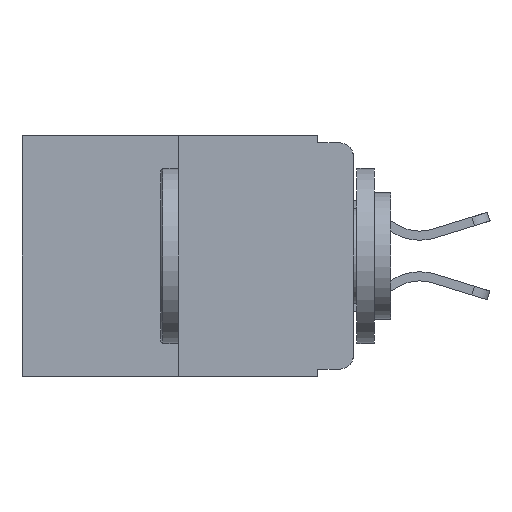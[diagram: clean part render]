
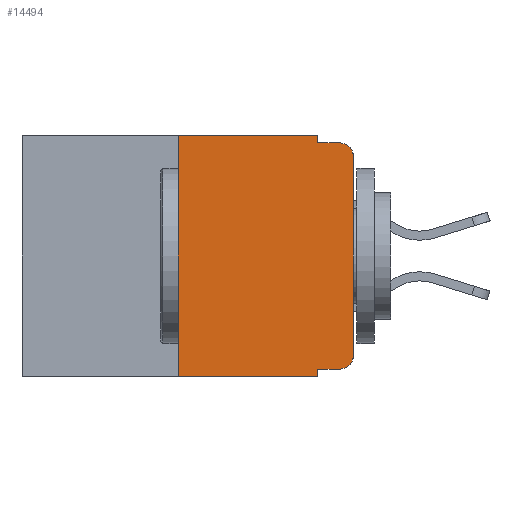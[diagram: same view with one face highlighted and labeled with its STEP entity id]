
A CAD part, left-side view. The second image highlights one B-rep face of the part: STEP entity #14494.
In plain terms, the highlighted planar face has unit normal (-1, 0, 0).
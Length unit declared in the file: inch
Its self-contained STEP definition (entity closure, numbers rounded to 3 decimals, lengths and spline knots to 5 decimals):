
#337 = CARTESIAN_POINT ( 'NONE',  ( 0., 0.473, 0. ) ) ;
#623 = DIRECTION ( 'NONE',  ( 0., -1., 0. ) ) ;
#686 = LINE ( 'NONE', #337, #7362 ) ;
#712 = EDGE_CURVE ( 'NONE', #9476, #1143, #9028, .T. ) ;
#891 = CARTESIAN_POINT ( 'NONE',  ( 0., 0.02, -0.03 ) ) ;
#1072 = VECTOR ( 'NONE', #5682, 39.37008 ) ;
#1143 = VERTEX_POINT ( 'NONE', #4148 ) ;
#1169 = CARTESIAN_POINT ( 'NONE',  ( 0., 0.051, 0. ) ) ;
#1214 = CARTESIAN_POINT ( 'NONE',  ( 0., 0.051, -0.333 ) ) ;
#1677 = CARTESIAN_POINT ( 'NONE',  ( 0., 0.473, 0. ) ) ;
#1696 = CIRCLE ( 'NONE', #11862, 0.02 ) ;
#1710 = DIRECTION ( 'NONE',  ( 0., 0., -1. ) ) ;
#2031 = LINE ( 'NONE', #1214, #5386 ) ;
#2071 = FACE_OUTER_BOUND ( 'NONE', #13560, .T. ) ;
#2201 = DIRECTION ( 'NONE',  ( 0., 0., -1. ) ) ;
#2268 = LINE ( 'NONE', #1169, #14534 ) ;
#2578 = ORIENTED_EDGE ( 'NONE', *, *, #15032, .F. ) ;
#2668 = ORIENTED_EDGE ( 'NONE', *, *, #10209, .F. ) ;
#2971 = DIRECTION ( 'NONE',  ( 1., 0., 0. ) ) ;
#2995 = AXIS2_PLACEMENT_3D ( 'NONE', #1677, #2971, #11547 ) ;
#3131 = LINE ( 'NONE', #15331, #12533 ) ;
#3512 = LINE ( 'NONE', #9941, #9684 ) ;
#3581 = VECTOR ( 'NONE', #1710, 39.37008 ) ;
#3655 = CARTESIAN_POINT ( 'NONE',  ( 0., 0., 0. ) ) ;
#3777 = CARTESIAN_POINT ( 'NONE',  ( 0., 0.02, -0.313 ) ) ;
#3823 = EDGE_CURVE ( 'NONE', #13723, #4353, #3512, .T. ) ;
#4036 = ORIENTED_EDGE ( 'NONE', *, *, #3823, .T. ) ;
#4148 = CARTESIAN_POINT ( 'NONE',  ( 0., 0., -0.03 ) ) ;
#4149 = CARTESIAN_POINT ( 'NONE',  ( 0., 0.02, -0.333 ) ) ;
#4353 = VERTEX_POINT ( 'NONE', #8444 ) ;
#4400 = DIRECTION ( 'NONE',  ( 0., 0., 1. ) ) ;
#5068 = DIRECTION ( 'NONE',  ( 0., 0., -1. ) ) ;
#5225 = CARTESIAN_POINT ( 'NONE',  ( 0., 0.051, -0.01 ) ) ;
#5386 = VECTOR ( 'NONE', #8688, 39.37008 ) ;
#5519 = ORIENTED_EDGE ( 'NONE', *, *, #15800, .T. ) ;
#5682 = DIRECTION ( 'NONE',  ( 0., 0., 1. ) ) ;
#5782 = VECTOR ( 'NONE', #4400, 39.37008 ) ;
#7362 = VECTOR ( 'NONE', #10311, 39.37008 ) ;
#7372 = CARTESIAN_POINT ( 'NONE',  ( 0., 0.25, 0. ) ) ;
#7411 = DIRECTION ( 'NONE',  ( 0., 0., -1. ) ) ;
#7618 = ORIENTED_EDGE ( 'NONE', *, *, #712, .T. ) ;
#7708 = CARTESIAN_POINT ( 'NONE',  ( 0., 0.051, 0. ) ) ;
#8290 = CARTESIAN_POINT ( 'NONE',  ( 0., 0.051, -0.333 ) ) ;
#8444 = CARTESIAN_POINT ( 'NONE',  ( 0., 0.051, -0.343 ) ) ;
#8580 = EDGE_CURVE ( 'NONE', #12487, #9476, #11610, .T. ) ;
#8649 = VERTEX_POINT ( 'NONE', #5225 ) ;
#8688 = DIRECTION ( 'NONE',  ( 0., -1., 0. ) ) ;
#9028 = LINE ( 'NONE', #3655, #5782 ) ;
#9127 = PLANE ( 'NONE',  #2995 ) ;
#9400 = EDGE_CURVE ( 'NONE', #10402, #12487, #2031, .T. ) ;
#9476 = VERTEX_POINT ( 'NONE', #14814 ) ;
#9547 = AXIS2_PLACEMENT_3D ( 'NONE', #3777, #12351, #5068 ) ;
#9614 = DIRECTION ( 'NONE',  ( -1., 0., 0. ) ) ;
#9684 = VECTOR ( 'NONE', #11150, 39.37008 ) ;
#9941 = CARTESIAN_POINT ( 'NONE',  ( 0., 0.473, -0.343 ) ) ;
#10066 = VERTEX_POINT ( 'NONE', #7708 ) ;
#10125 = LINE ( 'NONE', #11577, #3581 ) ;
#10209 = EDGE_CURVE ( 'NONE', #10402, #4353, #10125, .T. ) ;
#10311 = DIRECTION ( 'NONE',  ( 0., -1., 0. ) ) ;
#10402 = VERTEX_POINT ( 'NONE', #8290 ) ;
#11150 = DIRECTION ( 'NONE',  ( 0., -1., 0. ) ) ;
#11343 = ORIENTED_EDGE ( 'NONE', *, *, #9400, .T. ) ;
#11350 = LINE ( 'NONE', #14132, #1072 ) ;
#11468 = ORIENTED_EDGE ( 'NONE', *, *, #14267, .F. ) ;
#11547 = DIRECTION ( 'NONE',  ( 0., 0., -1. ) ) ;
#11577 = CARTESIAN_POINT ( 'NONE',  ( 0., 0.051, 0. ) ) ;
#11610 = CIRCLE ( 'NONE', #9547, 0.02 ) ;
#11862 = AXIS2_PLACEMENT_3D ( 'NONE', #891, #9614, #2201 ) ;
#11865 = ORIENTED_EDGE ( 'NONE', *, *, #13085, .F. ) ;
#12243 = ORIENTED_EDGE ( 'NONE', *, *, #13473, .F. ) ;
#12351 = DIRECTION ( 'NONE',  ( -1., 0., 0. ) ) ;
#12487 = VERTEX_POINT ( 'NONE', #4149 ) ;
#12533 = VECTOR ( 'NONE', #623, 39.37008 ) ;
#12839 = VERTEX_POINT ( 'NONE', #7372 ) ;
#13085 = EDGE_CURVE ( 'NONE', #12839, #10066, #686, .T. ) ;
#13473 = EDGE_CURVE ( 'NONE', #13723, #12839, #11350, .T. ) ;
#13560 = EDGE_LOOP ( 'NONE', ( #7618, #5519, #2578, #11468, #11865, #12243, #4036, #2668, #11343, #15260 ) ) ;
#13633 = VERTEX_POINT ( 'NONE', #14686 ) ;
#13723 = VERTEX_POINT ( 'NONE', #14842 ) ;
#14132 = CARTESIAN_POINT ( 'NONE',  ( 0., 0.25, 0. ) ) ;
#14267 = EDGE_CURVE ( 'NONE', #10066, #8649, #2268, .T. ) ;
#14494 = ADVANCED_FACE ( 'NONE', ( #2071 ), #9127, .F. ) ;
#14534 = VECTOR ( 'NONE', #7411, 39.37008 ) ;
#14686 = CARTESIAN_POINT ( 'NONE',  ( 0., 0.02, -0.01 ) ) ;
#14814 = CARTESIAN_POINT ( 'NONE',  ( 0., 0., -0.313 ) ) ;
#14842 = CARTESIAN_POINT ( 'NONE',  ( 0., 0.25, -0.343 ) ) ;
#15032 = EDGE_CURVE ( 'NONE', #8649, #13633, #3131, .T. ) ;
#15260 = ORIENTED_EDGE ( 'NONE', *, *, #8580, .T. ) ;
#15331 = CARTESIAN_POINT ( 'NONE',  ( 0., 0.051, -0.01 ) ) ;
#15800 = EDGE_CURVE ( 'NONE', #1143, #13633, #1696, .T. ) ;
